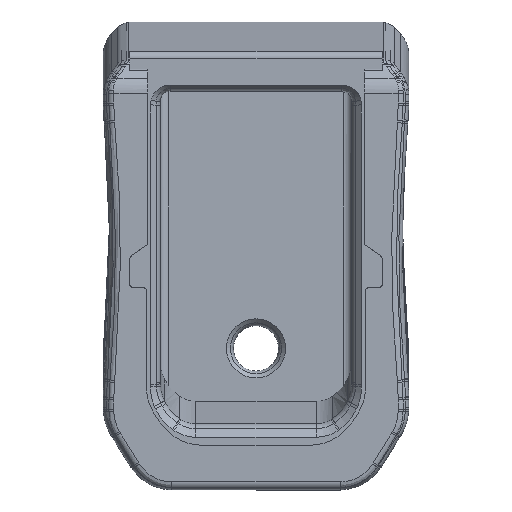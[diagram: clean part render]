
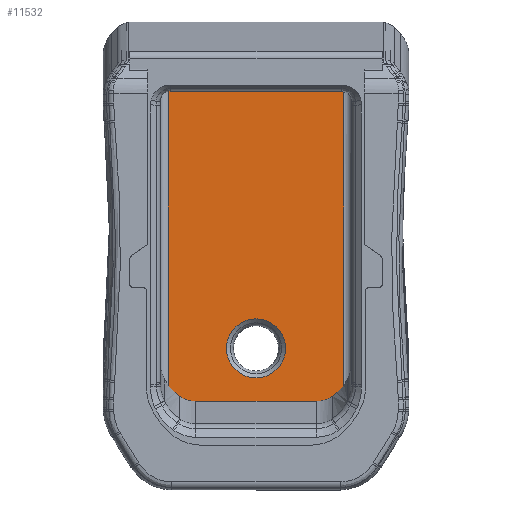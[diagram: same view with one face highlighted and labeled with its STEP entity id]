
A CAD part, top view. The second image highlights one B-rep face of the part: STEP entity #11532.
In plain terms, the highlighted planar face has unit normal (0, 0, 1).
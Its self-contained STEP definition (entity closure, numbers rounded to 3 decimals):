
#1361=ELLIPSE('',#12342,3.106,3.);
#1362=ELLIPSE('',#12343,3.106,3.);
#1363=ELLIPSE('',#12345,0.207,0.2);
#1364=ELLIPSE('',#12346,0.207,0.2);
#1440=LINE('',#15421,#1899);
#1441=LINE('',#15427,#1900);
#1442=LINE('',#15433,#1901);
#1443=LINE('',#15437,#1902);
#1899=VECTOR('',#13238,10.);
#1900=VECTOR('',#13243,10.);
#1901=VECTOR('',#13248,10.);
#1902=VECTOR('',#13251,10.);
#2499=FACE_BOUND('',#3384,.T.);
#2507=PLANE('',#12340);
#2604=FACE_OUTER_BOUND('',#3383,.T.);
#3383=EDGE_LOOP('',(#7750,#7751,#7752,#7753,#7754,#7755,#7756,#7757,#7758,
#7759));
#3384=EDGE_LOOP('',(#7760));
#4171=CIRCLE('',#12333,3.02);
#4176=CIRCLE('',#12341,4.599);
#4177=CIRCLE('',#12344,4.599);
#4706=VERTEX_POINT('',#15405);
#4710=VERTEX_POINT('',#15419);
#4711=VERTEX_POINT('',#15420);
#4712=VERTEX_POINT('',#15422);
#4713=VERTEX_POINT('',#15424);
#4714=VERTEX_POINT('',#15426);
#4715=VERTEX_POINT('',#15428);
#4716=VERTEX_POINT('',#15430);
#4717=VERTEX_POINT('',#15432);
#4718=VERTEX_POINT('',#15434);
#4719=VERTEX_POINT('',#15436);
#5835=EDGE_CURVE('',#4706,#4706,#4171,.T.);
#5841=EDGE_CURVE('',#4710,#4711,#1440,.T.);
#5842=EDGE_CURVE('',#4710,#4712,#4176,.F.);
#5843=EDGE_CURVE('',#4712,#4713,#1361,.F.);
#5844=EDGE_CURVE('',#4713,#4714,#1441,.F.);
#5845=EDGE_CURVE('',#4715,#4714,#1362,.T.);
#5846=EDGE_CURVE('',#4716,#4715,#4177,.T.);
#5847=EDGE_CURVE('',#4717,#4716,#1442,.T.);
#5848=EDGE_CURVE('',#4718,#4717,#1363,.T.);
#5849=EDGE_CURVE('',#4719,#4718,#1443,.T.);
#5850=EDGE_CURVE('',#4711,#4719,#1364,.T.);
#7750=ORIENTED_EDGE('',*,*,#5841,.F.);
#7751=ORIENTED_EDGE('',*,*,#5842,.T.);
#7752=ORIENTED_EDGE('',*,*,#5843,.T.);
#7753=ORIENTED_EDGE('',*,*,#5844,.T.);
#7754=ORIENTED_EDGE('',*,*,#5845,.F.);
#7755=ORIENTED_EDGE('',*,*,#5846,.F.);
#7756=ORIENTED_EDGE('',*,*,#5847,.F.);
#7757=ORIENTED_EDGE('',*,*,#5848,.F.);
#7758=ORIENTED_EDGE('',*,*,#5849,.F.);
#7759=ORIENTED_EDGE('',*,*,#5850,.F.);
#7760=ORIENTED_EDGE('',*,*,#5835,.F.);
#11532=ADVANCED_FACE('',(#2604,#2499),#2507,.T.);
#12333=AXIS2_PLACEMENT_3D('',#15407,#13221,#13222);
#12340=AXIS2_PLACEMENT_3D('',#15418,#13236,#13237);
#12341=AXIS2_PLACEMENT_3D('',#15423,#13239,#13240);
#12342=AXIS2_PLACEMENT_3D('',#15425,#13241,#13242);
#12343=AXIS2_PLACEMENT_3D('',#15429,#13244,#13245);
#12344=AXIS2_PLACEMENT_3D('',#15431,#13246,#13247);
#12345=AXIS2_PLACEMENT_3D('',#15435,#13249,#13250);
#12346=AXIS2_PLACEMENT_3D('',#15438,#13252,#13253);
#13221=DIRECTION('center_axis',(0.,0.,
1.));
#13222=DIRECTION('ref_axis',(-1.,0.,0.));
#13236=DIRECTION('center_axis',(0.,0.,
1.));
#13237=DIRECTION('ref_axis',(0.,-1.,0.));
#13238=DIRECTION('',(0.,1.,0.));
#13239=DIRECTION('center_axis',(0.,0.,
-1.));
#13240=DIRECTION('ref_axis',(1.,0.,0.));
#13241=DIRECTION('center_axis',(0.,0.,
-1.));
#13242=DIRECTION('ref_axis',(0.,-1.,0.));
#13243=DIRECTION('',(-1.,0.,0.));
#13244=DIRECTION('center_axis',(0.,0.,
-1.));
#13245=DIRECTION('ref_axis',(0.,-1.,0.));
#13246=DIRECTION('center_axis',(0.,0.,
-1.));
#13247=DIRECTION('ref_axis',(-1.,0.,0.));
#13248=DIRECTION('',(0.,-1.,0.));
#13249=DIRECTION('center_axis',(0.,0.,
-1.));
#13250=DIRECTION('ref_axis',(0.,1.,0.));
#13251=DIRECTION('',(1.,0.,0.));
#13252=DIRECTION('center_axis',(0.,0.,
-1.));
#13253=DIRECTION('ref_axis',(0.,1.,0.));
#15405=CARTESIAN_POINT('',(26.942,-26.718,-7.149));
#15407=CARTESIAN_POINT('Origin',(23.922,-26.718,-7.149));
#15418=CARTESIAN_POINT('Origin',(23.922,-17.523,-7.149));
#15419=CARTESIAN_POINT('',(14.924,-30.473,-7.149));
#15420=CARTESIAN_POINT('',(14.924,0.655,-7.149));
#15421=CARTESIAN_POINT('',(14.924,-24.313,-7.149));
#15422=CARTESIAN_POINT('',(16.081,-31.62,-7.149));
#15423=CARTESIAN_POINT('Origin',(18.689,-27.831,-7.149));
#15424=CARTESIAN_POINT('',(17.732,-32.139,-7.149));
#15425=CARTESIAN_POINT('Origin',(17.742,-29.033,-7.149));
#15426=CARTESIAN_POINT('',(30.112,-32.139,-7.149));
#15427=CARTESIAN_POINT('',(20.827,-32.139,-7.149));
#15428=CARTESIAN_POINT('',(31.763,-31.62,-7.149));
#15429=CARTESIAN_POINT('Origin',(30.102,-29.033,-7.149));
#15430=CARTESIAN_POINT('',(32.92,-30.473,-7.149));
#15431=CARTESIAN_POINT('Origin',(29.156,-27.831,-7.149));
#15432=CARTESIAN_POINT('',(32.92,0.655,-7.149));
#15433=CARTESIAN_POINT('',(32.92,-24.313,-7.149));
#15434=CARTESIAN_POINT('',(32.72,0.862,-7.149));
#15435=CARTESIAN_POINT('Origin',(32.72,0.655,-7.149));
#15436=CARTESIAN_POINT('',(15.124,0.862,-7.149));
#15437=CARTESIAN_POINT('',(19.745,0.862,-7.149));
#15438=CARTESIAN_POINT('Origin',(15.124,0.655,-7.149));
